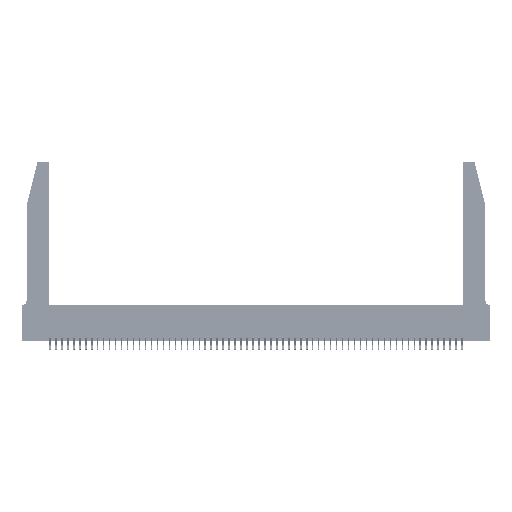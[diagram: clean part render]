
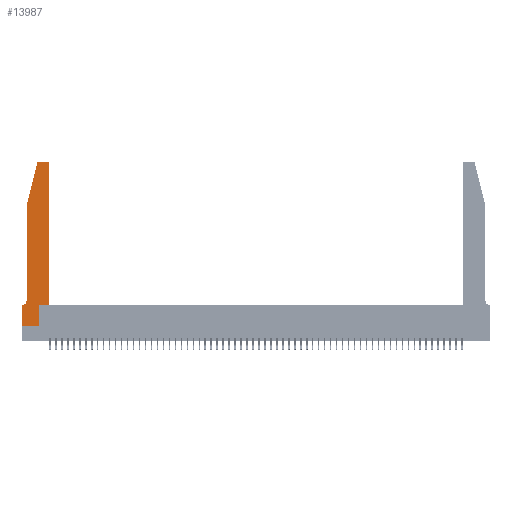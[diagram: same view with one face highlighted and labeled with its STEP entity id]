
A CAD part, top view. The second image highlights one B-rep face of the part: STEP entity #13987.
In plain terms, the highlighted planar face has unit normal (0, 0, 1).
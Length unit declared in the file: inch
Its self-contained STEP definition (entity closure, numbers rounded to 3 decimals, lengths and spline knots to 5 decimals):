
#89 = CARTESIAN_POINT ( 'NONE',  ( 0., 0.35, 0.37 ) ) ;
#161 = CARTESIAN_POINT ( 'NONE',  ( 0.4505, 0.35, 0.37 ) ) ;
#787 = EDGE_CURVE ( 'NONE', #46968, #36084, #14843, .T. ) ;
#1143 = CARTESIAN_POINT ( 'NONE',  ( 0.2605, 2.75, 0.37 ) ) ;
#1286 = VERTEX_POINT ( 'NONE', #89 ) ;
#1472 = CARTESIAN_POINT ( 'NONE',  ( 0.2865, 0., 0.37 ) ) ;
#1909 = DIRECTION ( 'NONE',  ( 0., 0., 1. ) ) ;
#3181 = ORIENTED_EDGE ( 'NONE', *, *, #7966, .T. ) ;
#3616 = DIRECTION ( 'NONE',  ( 1., 0., 0. ) ) ;
#4141 = VECTOR ( 'NONE', #41083, 39.37008 ) ;
#5104 = AXIS2_PLACEMENT_3D ( 'NONE', #5553, #35878, #9957 ) ;
#5359 = ORIENTED_EDGE ( 'NONE', *, *, #9967, .T. ) ;
#5553 = CARTESIAN_POINT ( 'NONE',  ( 0.284, 2.72, 0.37 ) ) ;
#5936 = VERTEX_POINT ( 'NONE', #15194 ) ;
#6111 = VERTEX_POINT ( 'NONE', #20639 ) ;
#7774 = AXIS2_PLACEMENT_3D ( 'NONE', #12130, #42420, #16467 ) ;
#7945 = VECTOR ( 'NONE', #30075, 39.37008 ) ;
#7966 = EDGE_CURVE ( 'NONE', #42632, #19557, #49329, .T. ) ;
#8126 = LINE ( 'NONE', #29520, #49267 ) ;
#9875 = DIRECTION ( 'NONE',  ( 0., -1., 0. ) ) ;
#9925 = DIRECTION ( 'NONE',  ( -1., 0., 0. ) ) ;
#9957 = DIRECTION ( 'NONE',  ( 1., 0., 0. ) ) ;
#9967 = EDGE_CURVE ( 'NONE', #19557, #46968, #32115, .T. ) ;
#10438 = VECTOR ( 'NONE', #3616, 39.37008 ) ;
#11187 = ORIENTED_EDGE ( 'NONE', *, *, #49678, .T. ) ;
#11261 = VECTOR ( 'NONE', #9875, 39.37008 ) ;
#12130 = CARTESIAN_POINT ( 'NONE',  ( 0.4205, 2.72, 0.37 ) ) ;
#13290 = VECTOR ( 'NONE', #28831, 39.37008 ) ;
#13316 = DIRECTION ( 'NONE',  ( 0., 1., 0. ) ) ;
#13528 = VERTEX_POINT ( 'NONE', #37819 ) ;
#13987 = ADVANCED_FACE ( 'NONE', ( #40686 ), #23553, .T. ) ;
#14639 = LINE ( 'NONE', #24492, #13290 ) ;
#14732 = VECTOR ( 'NONE', #13316, 39.37008 ) ;
#14843 = LINE ( 'NONE', #1143, #36531 ) ;
#15194 = CARTESIAN_POINT ( 'NONE',  ( 0.25487, 2.72718, 0.37 ) ) ;
#15625 = ORIENTED_EDGE ( 'NONE', *, *, #787, .T. ) ;
#16467 = DIRECTION ( 'NONE',  ( 1., 0., 0. ) ) ;
#17006 = EDGE_CURVE ( 'NONE', #13528, #32118, #55398, .T. ) ;
#17636 = EDGE_CURVE ( 'NONE', #36084, #5936, #35680, .T. ) ;
#17885 = EDGE_CURVE ( 'NONE', #6111, #42632, #14639, .T. ) ;
#18345 = VERTEX_POINT ( 'NONE', #1472 ) ;
#19029 = CARTESIAN_POINT ( 'NONE',  ( 0.284, 2.75, 0.37 ) ) ;
#19557 = VERTEX_POINT ( 'NONE', #27717 ) ;
#20592 = ORIENTED_EDGE ( 'NONE', *, *, #37295, .T. ) ;
#20639 = CARTESIAN_POINT ( 'NONE',  ( 0.2865, 0.35, 0.37 ) ) ;
#20811 = VECTOR ( 'NONE', #53537, 39.37008 ) ;
#23553 = PLANE ( 'NONE',  #46060 ) ;
#24131 = CARTESIAN_POINT ( 'NONE',  ( 0.0055, 0.42, 0.37 ) ) ;
#24171 = ORIENTED_EDGE ( 'NONE', *, *, #55123, .T. ) ;
#24492 = CARTESIAN_POINT ( 'NONE',  ( 0.4505, 0.35, 0.37 ) ) ;
#26009 = CIRCLE ( 'NONE', #32927, 0.07 ) ;
#26480 = ORIENTED_EDGE ( 'NONE', *, *, #42668, .T. ) ;
#26856 = EDGE_CURVE ( 'NONE', #53762, #18345, #55133, .T. ) ;
#27717 = CARTESIAN_POINT ( 'NONE',  ( 0.4505, 2.72, 0.37 ) ) ;
#28476 = DIRECTION ( 'NONE',  ( -1., 0., 0. ) ) ;
#28831 = DIRECTION ( 'NONE',  ( 1., 0., 0. ) ) ;
#29410 = CARTESIAN_POINT ( 'NONE',  ( 0., 0., 0.37 ) ) ;
#29520 = CARTESIAN_POINT ( 'NONE',  ( 0.2865, 0.35, 0.37 ) ) ;
#30075 = DIRECTION ( 'NONE',  ( -1., 0., 0. ) ) ;
#30660 = CARTESIAN_POINT ( 'NONE',  ( 0.4205, 2.75, 0.37 ) ) ;
#32115 = CIRCLE ( 'NONE', #7774, 0.03 ) ;
#32118 = VERTEX_POINT ( 'NONE', #46554 ) ;
#32250 = DIRECTION ( 'NONE',  ( 1., 0., 0. ) ) ;
#32927 = AXIS2_PLACEMENT_3D ( 'NONE', #24131, #54424, #28476 ) ;
#35014 = ORIENTED_EDGE ( 'NONE', *, *, #17636, .T. ) ;
#35680 = CIRCLE ( 'NONE', #5104, 0.03 ) ;
#35808 = CARTESIAN_POINT ( 'NONE',  ( 0.4505, 0.35, 0.37 ) ) ;
#35878 = DIRECTION ( 'NONE',  ( 0., 0., 1. ) ) ;
#36084 = VERTEX_POINT ( 'NONE', #19029 ) ;
#36531 = VECTOR ( 'NONE', #9925, 39.37008 ) ;
#36766 = VERTEX_POINT ( 'NONE', #48162 ) ;
#37295 = EDGE_CURVE ( 'NONE', #36766, #1286, #54016, .T. ) ;
#37819 = CARTESIAN_POINT ( 'NONE',  ( 0.0755, 2., 0.37 ) ) ;
#38282 = CARTESIAN_POINT ( 'NONE',  ( 0., 0., 0.37 ) ) ;
#40686 = FACE_OUTER_BOUND ( 'NONE', #54926, .T. ) ;
#41083 = DIRECTION ( 'NONE',  ( -0.239, -0.971, 0. ) ) ;
#42361 = EDGE_CURVE ( 'NONE', #18345, #6111, #8126, .T. ) ;
#42420 = DIRECTION ( 'NONE',  ( 0., 0., 1. ) ) ;
#42632 = VERTEX_POINT ( 'NONE', #35808 ) ;
#42668 = EDGE_CURVE ( 'NONE', #1286, #53762, #55954, .T. ) ;
#44050 = ORIENTED_EDGE ( 'NONE', *, *, #17006, .T. ) ;
#44854 = CARTESIAN_POINT ( 'NONE',  ( 0.0755, 2., 0.37 ) ) ;
#46060 = AXIS2_PLACEMENT_3D ( 'NONE', #53851, #1909, #32250 ) ;
#46554 = CARTESIAN_POINT ( 'NONE',  ( 0.0755, 0.42, 0.37 ) ) ;
#46968 = VERTEX_POINT ( 'NONE', #30660 ) ;
#48051 = ORIENTED_EDGE ( 'NONE', *, *, #17885, .T. ) ;
#48162 = CARTESIAN_POINT ( 'NONE',  ( 0.0055, 0.35, 0.37 ) ) ;
#49076 = CARTESIAN_POINT ( 'NONE',  ( 0., 0., 0.37 ) ) ;
#49267 = VECTOR ( 'NONE', #55275, 39.37008 ) ;
#49329 = LINE ( 'NONE', #161, #14732 ) ;
#49678 = EDGE_CURVE ( 'NONE', #5936, #13528, #50276, .T. ) ;
#49795 = CARTESIAN_POINT ( 'NONE',  ( 0.0755, 2., 0.37 ) ) ;
#50276 = LINE ( 'NONE', #49795, #4141 ) ;
#50322 = ORIENTED_EDGE ( 'NONE', *, *, #42361, .T. ) ;
#51693 = CARTESIAN_POINT ( 'NONE',  ( 0.0755, 0.35, 0.37 ) ) ;
#53220 = ORIENTED_EDGE ( 'NONE', *, *, #26856, .T. ) ;
#53537 = DIRECTION ( 'NONE',  ( 0., -1., 0. ) ) ;
#53762 = VERTEX_POINT ( 'NONE', #38282 ) ;
#53851 = CARTESIAN_POINT ( 'NONE',  ( 0., 0.35, 0.37 ) ) ;
#54016 = LINE ( 'NONE', #51693, #7945 ) ;
#54424 = DIRECTION ( 'NONE',  ( 0., 0., -1. ) ) ;
#54926 = EDGE_LOOP ( 'NONE', ( #15625, #35014, #11187, #44050, #24171, #20592, #26480, #53220, #50322, #48051, #3181, #5359 ) ) ;
#55123 = EDGE_CURVE ( 'NONE', #32118, #36766, #26009, .T. ) ;
#55133 = LINE ( 'NONE', #29410, #10438 ) ;
#55275 = DIRECTION ( 'NONE',  ( 0., 1., 0. ) ) ;
#55398 = LINE ( 'NONE', #44854, #20811 ) ;
#55954 = LINE ( 'NONE', #49076, #11261 ) ;
